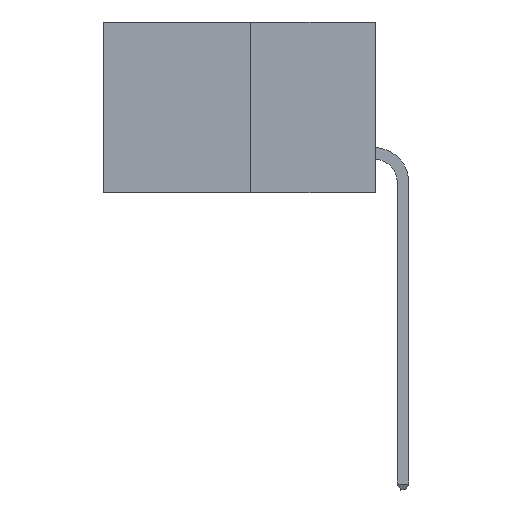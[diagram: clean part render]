
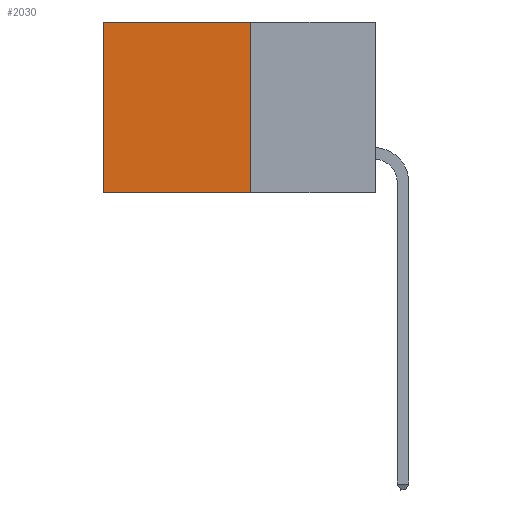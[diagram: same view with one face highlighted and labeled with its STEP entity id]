
A CAD part, left-side view. The second image highlights one B-rep face of the part: STEP entity #2030.
In plain terms, the highlighted planar face has unit normal (-1, 0, 0).
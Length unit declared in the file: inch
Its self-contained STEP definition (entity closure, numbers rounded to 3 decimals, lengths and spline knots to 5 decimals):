
#685 = DIRECTION ( 'NONE',  ( 0., 1., 0. ) ) ;
#1376 = CARTESIAN_POINT ( 'NONE',  ( 0.277, 0.59, 0. ) ) ;
#1498 = EDGE_LOOP ( 'NONE', ( #2505, #7850, #8624, #3208 ) ) ;
#1816 = VECTOR ( 'NONE', #9899, 39.37008 ) ;
#2002 = VECTOR ( 'NONE', #685, 39.37008 ) ;
#2030 = ADVANCED_FACE ( 'NONE', ( #4023 ), #6039, .F. ) ;
#2259 = LINE ( 'NONE', #6348, #2002 ) ;
#2393 = EDGE_CURVE ( 'NONE', #5621, #2777, #6627, .T. ) ;
#2497 = CARTESIAN_POINT ( 'NONE',  ( 0.277, 0.27, -0.37 ) ) ;
#2505 = ORIENTED_EDGE ( 'NONE', *, *, #2393, .T. ) ;
#2552 = DIRECTION ( 'NONE',  ( 0., 0., -1. ) ) ;
#2611 = VECTOR ( 'NONE', #2552, 39.37008 ) ;
#2777 = VERTEX_POINT ( 'NONE', #8973 ) ;
#3113 = EDGE_CURVE ( 'NONE', #4150, #9847, #4524, .T. ) ;
#3208 = ORIENTED_EDGE ( 'NONE', *, *, #7513, .T. ) ;
#4023 = FACE_OUTER_BOUND ( 'NONE', #1498, .T. ) ;
#4150 = VERTEX_POINT ( 'NONE', #5014 ) ;
#4523 = VECTOR ( 'NONE', #8567, 39.37008 ) ;
#4524 = LINE ( 'NONE', #2497, #2611 ) ;
#4770 = DIRECTION ( 'NONE',  ( 0., 0., -1. ) ) ;
#4786 = DIRECTION ( 'NONE',  ( 1., 0., 0. ) ) ;
#5014 = CARTESIAN_POINT ( 'NONE',  ( 0.277, 0.27, 0. ) ) ;
#5110 = EDGE_CURVE ( 'NONE', #9847, #2777, #2259, .T. ) ;
#5255 = CARTESIAN_POINT ( 'NONE',  ( 0.277, 0.27, -0.37 ) ) ;
#5318 = CARTESIAN_POINT ( 'NONE',  ( 0.277, 0.27, 0. ) ) ;
#5621 = VERTEX_POINT ( 'NONE', #1376 ) ;
#6039 = PLANE ( 'NONE',  #6584 ) ;
#6348 = CARTESIAN_POINT ( 'NONE',  ( 0.277, 0.27, -0.37 ) ) ;
#6584 = AXIS2_PLACEMENT_3D ( 'NONE', #5255, #4786, #4770 ) ;
#6627 = LINE ( 'NONE', #8245, #4523 ) ;
#6628 = CARTESIAN_POINT ( 'NONE',  ( 0.277, 0.27, -0.37 ) ) ;
#7513 = EDGE_CURVE ( 'NONE', #4150, #5621, #7940, .T. ) ;
#7850 = ORIENTED_EDGE ( 'NONE', *, *, #5110, .F. ) ;
#7940 = LINE ( 'NONE', #5318, #1816 ) ;
#8245 = CARTESIAN_POINT ( 'NONE',  ( 0.277, 0.59, -0.37 ) ) ;
#8567 = DIRECTION ( 'NONE',  ( 0., 0., -1. ) ) ;
#8624 = ORIENTED_EDGE ( 'NONE', *, *, #3113, .F. ) ;
#8973 = CARTESIAN_POINT ( 'NONE',  ( 0.277, 0.59, -0.37 ) ) ;
#9847 = VERTEX_POINT ( 'NONE', #6628 ) ;
#9899 = DIRECTION ( 'NONE',  ( 0., 1., 0. ) ) ;
